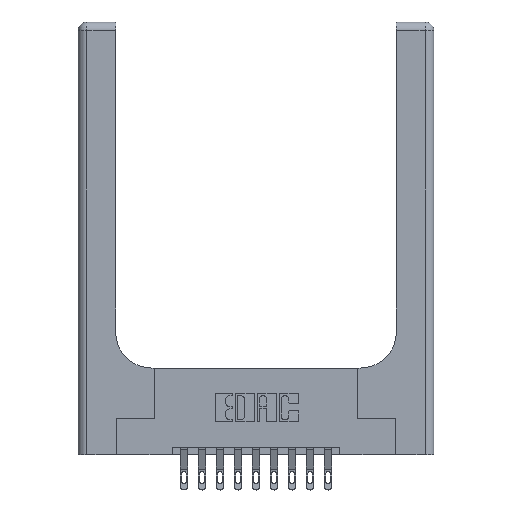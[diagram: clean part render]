
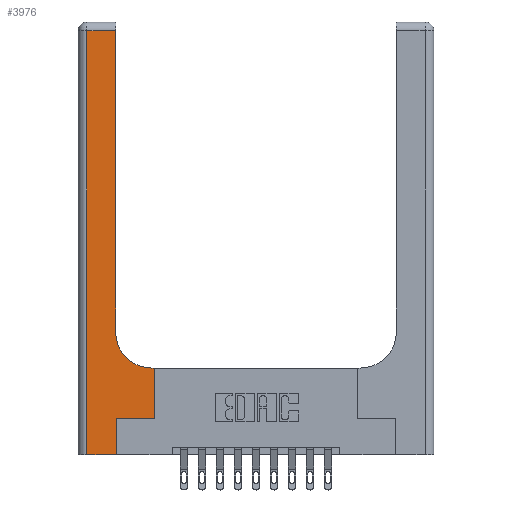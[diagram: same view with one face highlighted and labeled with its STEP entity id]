
A CAD part, top view. The second image highlights one B-rep face of the part: STEP entity #3976.
In plain terms, the highlighted planar face has unit normal (0, 0, 1).
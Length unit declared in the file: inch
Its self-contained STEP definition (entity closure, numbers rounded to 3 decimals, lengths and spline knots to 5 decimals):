
#30 = LINE ( 'NONE', #5188, #9120 ) ;
#220 = CARTESIAN_POINT ( 'NONE',  ( 0.528, 0.25, 0.37 ) ) ;
#384 = CARTESIAN_POINT ( 'NONE',  ( 0.06, 2.94, 0.37 ) ) ;
#401 = DIRECTION ( 'NONE',  ( 1., 0., 0. ) ) ;
#433 = VERTEX_POINT ( 'NONE', #6393 ) ;
#791 = CARTESIAN_POINT ( 'NONE',  ( 0.528, 0.6, 0.37 ) ) ;
#1037 = ORIENTED_EDGE ( 'NONE', *, *, #8752, .T. ) ;
#1096 = DIRECTION ( 'NONE',  ( 1., 0., 0. ) ) ;
#1137 = ORIENTED_EDGE ( 'NONE', *, *, #5860, .T. ) ;
#1822 = VECTOR ( 'NONE', #13819, 39.37008 ) ;
#1859 = VECTOR ( 'NONE', #9175, 39.37008 ) ;
#1975 = LINE ( 'NONE', #2052, #6704 ) ;
#2052 = CARTESIAN_POINT ( 'NONE',  ( 0.265, 0.25, 0.37 ) ) ;
#2074 = DIRECTION ( 'NONE',  ( 1., 0., 0. ) ) ;
#2078 = ORIENTED_EDGE ( 'NONE', *, *, #10133, .T. ) ;
#2423 = VERTEX_POINT ( 'NONE', #10641 ) ;
#3097 = CARTESIAN_POINT ( 'NONE',  ( 0.265, 0.25, 0.37 ) ) ;
#3226 = EDGE_CURVE ( 'NONE', #10829, #11899, #1975, .T. ) ;
#3409 = VECTOR ( 'NONE', #7918, 39.37008 ) ;
#3707 = CARTESIAN_POINT ( 'NONE',  ( 0.26, 3., 0.37 ) ) ;
#3907 = CARTESIAN_POINT ( 'NONE',  ( 0., 3., 0.37 ) ) ;
#3976 = ADVANCED_FACE ( 'NONE', ( #15032 ), #7544, .F. ) ;
#4142 = EDGE_LOOP ( 'NONE', ( #1037, #2078, #15770, #16073, #1137, #12147, #6197, #16049, #15045 ) ) ;
#4158 = CARTESIAN_POINT ( 'NONE',  ( 0., 2.94, 0.37 ) ) ;
#4523 = LINE ( 'NONE', #4682, #14792 ) ;
#4654 = EDGE_CURVE ( 'NONE', #2423, #5357, #4523, .T. ) ;
#4682 = CARTESIAN_POINT ( 'NONE',  ( 0., 0., 0.37 ) ) ;
#5188 = CARTESIAN_POINT ( 'NONE',  ( 0.26, 0.6, 0.37 ) ) ;
#5303 = DIRECTION ( 'NONE',  ( 0., -1., 0. ) ) ;
#5357 = VERTEX_POINT ( 'NONE', #7858 ) ;
#5716 = EDGE_CURVE ( 'NONE', #14451, #15476, #30, .T. ) ;
#5734 = CIRCLE ( 'NONE', #7862, 0.25 ) ;
#5860 = EDGE_CURVE ( 'NONE', #5357, #10829, #10452, .T. ) ;
#6197 = ORIENTED_EDGE ( 'NONE', *, *, #9538, .T. ) ;
#6393 = CARTESIAN_POINT ( 'NONE',  ( 0.26, 0.85, 0.37 ) ) ;
#6493 = CARTESIAN_POINT ( 'NONE',  ( 0.26, 2.94, 0.37 ) ) ;
#6538 = CARTESIAN_POINT ( 'NONE',  ( 0.06, 3., 0.37 ) ) ;
#6704 = VECTOR ( 'NONE', #401, 39.37008 ) ;
#7544 = PLANE ( 'NONE',  #12199 ) ;
#7858 = CARTESIAN_POINT ( 'NONE',  ( 0.265, 0., 0.37 ) ) ;
#7862 = AXIS2_PLACEMENT_3D ( 'NONE', #12371, #14760, #1096 ) ;
#7918 = DIRECTION ( 'NONE',  ( 0., 1., 0. ) ) ;
#8080 = DIRECTION ( 'NONE',  ( 0., 1., 0. ) ) ;
#8230 = LINE ( 'NONE', #9135, #3409 ) ;
#8702 = VECTOR ( 'NONE', #5303, 39.37008 ) ;
#8752 = EDGE_CURVE ( 'NONE', #433, #9416, #14894, .T. ) ;
#9120 = VECTOR ( 'NONE', #11212, 39.37008 ) ;
#9135 = CARTESIAN_POINT ( 'NONE',  ( 0.528, 0.25, 0.37 ) ) ;
#9144 = CARTESIAN_POINT ( 'NONE',  ( 0.265, 0., 0.37 ) ) ;
#9175 = DIRECTION ( 'NONE',  ( -1., 0., 0. ) ) ;
#9306 = EDGE_CURVE ( 'NONE', #15476, #433, #5734, .T. ) ;
#9416 = VERTEX_POINT ( 'NONE', #6493 ) ;
#9538 = EDGE_CURVE ( 'NONE', #11899, #14451, #8230, .T. ) ;
#9651 = VECTOR ( 'NONE', #8080, 39.37008 ) ;
#10083 = DIRECTION ( 'NONE',  ( 0., 0., -1. ) ) ;
#10133 = EDGE_CURVE ( 'NONE', #9416, #11901, #12801, .T. ) ;
#10452 = LINE ( 'NONE', #9144, #9651 ) ;
#10641 = CARTESIAN_POINT ( 'NONE',  ( 0.06, 0., 0.37 ) ) ;
#10648 = EDGE_CURVE ( 'NONE', #11901, #2423, #11569, .T. ) ;
#10829 = VERTEX_POINT ( 'NONE', #3097 ) ;
#11212 = DIRECTION ( 'NONE',  ( -1., 0., 0. ) ) ;
#11569 = LINE ( 'NONE', #6538, #8702 ) ;
#11899 = VERTEX_POINT ( 'NONE', #220 ) ;
#11901 = VERTEX_POINT ( 'NONE', #384 ) ;
#12147 = ORIENTED_EDGE ( 'NONE', *, *, #3226, .T. ) ;
#12199 = AXIS2_PLACEMENT_3D ( 'NONE', #3907, #10083, #15107 ) ;
#12371 = CARTESIAN_POINT ( 'NONE',  ( 0.51, 0.85, 0.37 ) ) ;
#12801 = LINE ( 'NONE', #4158, #1859 ) ;
#13140 = CARTESIAN_POINT ( 'NONE',  ( 0.51, 0.6, 0.37 ) ) ;
#13819 = DIRECTION ( 'NONE',  ( 0., 1., 0. ) ) ;
#14451 = VERTEX_POINT ( 'NONE', #791 ) ;
#14760 = DIRECTION ( 'NONE',  ( 0., 0., -1. ) ) ;
#14792 = VECTOR ( 'NONE', #2074, 39.37008 ) ;
#14894 = LINE ( 'NONE', #3707, #1822 ) ;
#15032 = FACE_OUTER_BOUND ( 'NONE', #4142, .T. ) ;
#15045 = ORIENTED_EDGE ( 'NONE', *, *, #9306, .T. ) ;
#15107 = DIRECTION ( 'NONE',  ( -1., 0., 0. ) ) ;
#15476 = VERTEX_POINT ( 'NONE', #13140 ) ;
#15770 = ORIENTED_EDGE ( 'NONE', *, *, #10648, .T. ) ;
#16049 = ORIENTED_EDGE ( 'NONE', *, *, #5716, .T. ) ;
#16073 = ORIENTED_EDGE ( 'NONE', *, *, #4654, .T. ) ;
